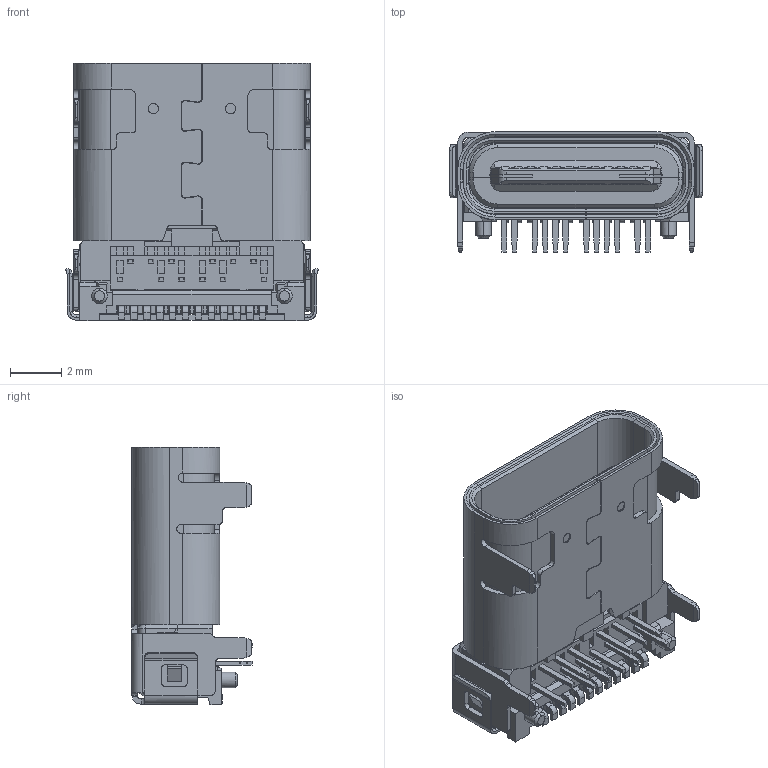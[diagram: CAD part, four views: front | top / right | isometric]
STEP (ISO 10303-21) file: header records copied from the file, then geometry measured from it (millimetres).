
FILE_DESCRIPTION (( 'STEP AP214' ), '1' );
FILE_NAME ('698C124-208-211.STEP', '2021-01-15T18:24:22', ( '' ), ( '' ), 'SwSTEP 2.0', 'SolidWorks 2020', '' );
FILE_SCHEMA (( 'AUTOMOTIVE_DESIGN' ));
Length unit declared in the file: millimetre
Products named in the file (4): Insulator1 698C124-X08-211; Shell 698C124-X08-211; 698C124-208-211; Insulator2 698C124-X08-211
Assembly tree (3 placements, depth 2):
  698C124-208-211
    Insulator2 698C124-X08-211
    Shell 698C124-X08-211
    Insulator1 698C124-X08-211
Bounding box: 9.83 x 4.68 x 10.03 mm (x, y, z)
Volume: 167.5 mm3; surface area: 1423.1 mm2
Topology: 3 solids, 27 shells, 3138 faces, 9403 edges, 6124 vertices
Faces by surface type: plane 2372, cylinder 671, cone 80, bspline 15
Entity records: 116235 total; most frequent: CARTESIAN_POINT 29335, ORIENTED_EDGE 18790, DIRECTION 13265, EDGE_CURVE 9395, LINE 6719, VECTOR 6719, VERTEX_POINT 6124, EDGE_LOOP 3295
